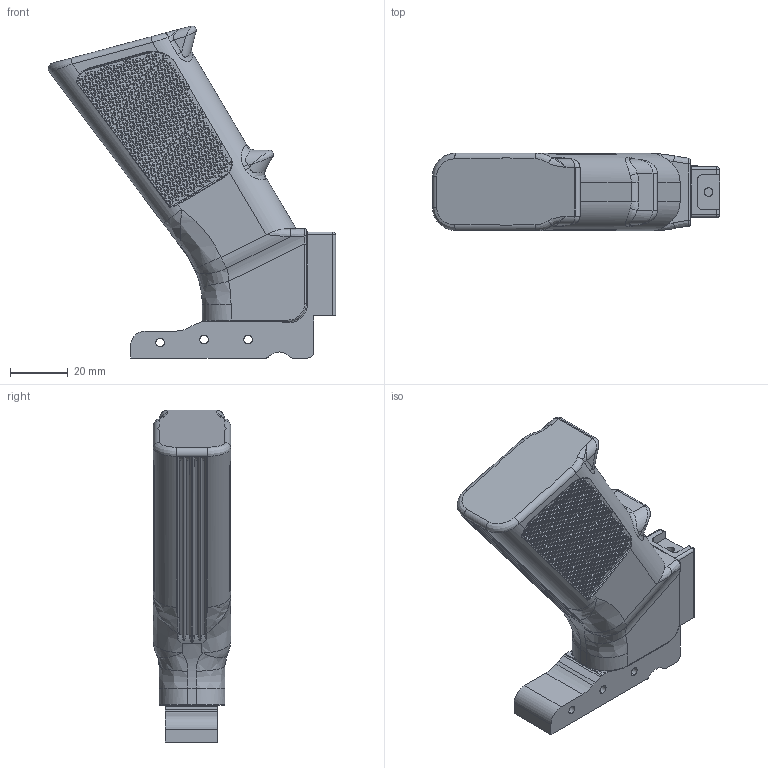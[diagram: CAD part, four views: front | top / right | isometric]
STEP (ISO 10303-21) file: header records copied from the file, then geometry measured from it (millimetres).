
FILE_DESCRIPTION (( 'STEP AP214' ), '1' );
FILE_NAME ('Thunderbolt_Pistol_Grip_Combo.STEP', '2021-09-12T03:53:34', ( '' ), ( '' ), 'SwSTEP 2.0', 'SolidWorks 2020', '' );
FILE_SCHEMA (( 'AUTOMOTIVE_DESIGN' ));
Products named in the file (1): Thunderbolt_Pistol_Grip_Combo
Bounding box: 99.34 x 26.8 x 114.8 mm (x, y, z)
Volume: 121457.8 mm3; surface area: 21419.5 mm2
Topology: 1 solids, 2 shells, 6272 faces, 12713 edges, 7932 vertices
Faces by surface type: plane 6064, cylinder 115, bspline 85, torus 6, sphere 2
Entity records: 166133 total; most frequent: CARTESIAN_POINT 41682, ORIENTED_EDGE 25404, DIRECTION 22014, EDGE_CURVE 12702, VECTOR 9278, LINE 9278, VERTEX_POINT 7932, EDGE_LOOP 7782
